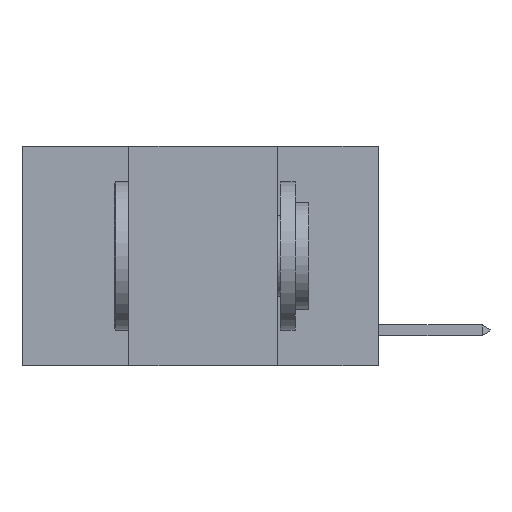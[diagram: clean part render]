
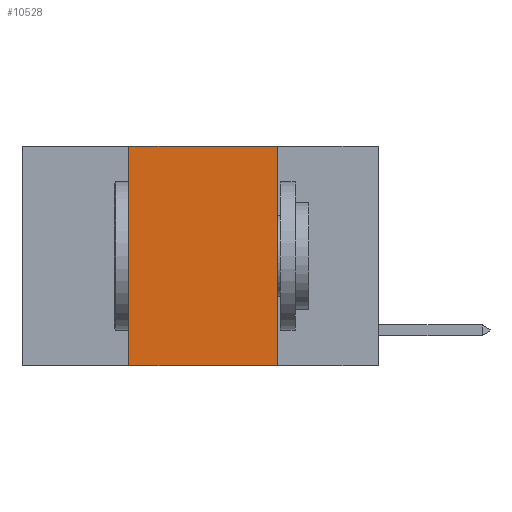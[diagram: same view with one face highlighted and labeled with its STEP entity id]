
A CAD part, left-side view. The second image highlights one B-rep face of the part: STEP entity #10528.
In plain terms, the highlighted planar face has unit normal (-1, 0, 0).
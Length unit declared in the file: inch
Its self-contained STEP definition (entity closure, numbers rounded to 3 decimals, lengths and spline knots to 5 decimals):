
#221 = FACE_OUTER_BOUND ( 'NONE', #9805, .T. ) ;
#280 = EDGE_CURVE ( 'NONE', #2071, #11001, #12341, .T. ) ;
#474 = CARTESIAN_POINT ( 'NONE',  ( 0., 0.42, 0. ) ) ;
#533 = CARTESIAN_POINT ( 'NONE',  ( 0., 0.6, 0. ) ) ;
#880 = CARTESIAN_POINT ( 'NONE',  ( 0., 0.6, -0.37 ) ) ;
#1016 = CARTESIAN_POINT ( 'NONE',  ( 0., 0.17, -0.37 ) ) ;
#1208 = ORIENTED_EDGE ( 'NONE', *, *, #8755, .F. ) ;
#1375 = LINE ( 'NONE', #10526, #2928 ) ;
#2071 = VERTEX_POINT ( 'NONE', #2213 ) ;
#2146 = ORIENTED_EDGE ( 'NONE', *, *, #280, .F. ) ;
#2213 = CARTESIAN_POINT ( 'NONE',  ( 0., 0.42, -0.37 ) ) ;
#2878 = VECTOR ( 'NONE', #5505, 39.37008 ) ;
#2928 = VECTOR ( 'NONE', #11551, 39.37008 ) ;
#3028 = VERTEX_POINT ( 'NONE', #1016 ) ;
#3667 = CARTESIAN_POINT ( 'NONE',  ( 0., 0.17, 0. ) ) ;
#3911 = LINE ( 'NONE', #880, #8127 ) ;
#4099 = VERTEX_POINT ( 'NONE', #3667 ) ;
#4782 = AXIS2_PLACEMENT_3D ( 'NONE', #6135, #7045, #6007 ) ;
#5131 = CARTESIAN_POINT ( 'NONE',  ( 0., 0.42, 0. ) ) ;
#5505 = DIRECTION ( 'NONE',  ( 0., -1., 0. ) ) ;
#6007 = DIRECTION ( 'NONE',  ( 0., 0., -1. ) ) ;
#6135 = CARTESIAN_POINT ( 'NONE',  ( 0., 0.6, 0. ) ) ;
#6690 = LINE ( 'NONE', #533, #2878 ) ;
#7045 = DIRECTION ( 'NONE',  ( 1., 0., 0. ) ) ;
#8067 = ORIENTED_EDGE ( 'NONE', *, *, #11141, .F. ) ;
#8127 = VECTOR ( 'NONE', #11596, 39.37008 ) ;
#8755 = EDGE_CURVE ( 'NONE', #11001, #4099, #6690, .T. ) ;
#9805 = EDGE_LOOP ( 'NONE', ( #8067, #1208, #2146, #12051 ) ) ;
#10192 = PLANE ( 'NONE',  #4782 ) ;
#10367 = EDGE_CURVE ( 'NONE', #2071, #3028, #3911, .T. ) ;
#10526 = CARTESIAN_POINT ( 'NONE',  ( 0., 0.17, 0. ) ) ;
#10528 = ADVANCED_FACE ( 'NONE', ( #221 ), #10192, .F. ) ;
#11001 = VERTEX_POINT ( 'NONE', #5131 ) ;
#11141 = EDGE_CURVE ( 'NONE', #4099, #3028, #1375, .T. ) ;
#11551 = DIRECTION ( 'NONE',  ( 0., 0., -1. ) ) ;
#11596 = DIRECTION ( 'NONE',  ( 0., -1., 0. ) ) ;
#11814 = VECTOR ( 'NONE', #12149, 39.37008 ) ;
#12051 = ORIENTED_EDGE ( 'NONE', *, *, #10367, .T. ) ;
#12149 = DIRECTION ( 'NONE',  ( 0., 0., 1. ) ) ;
#12341 = LINE ( 'NONE', #474, #11814 ) ;
